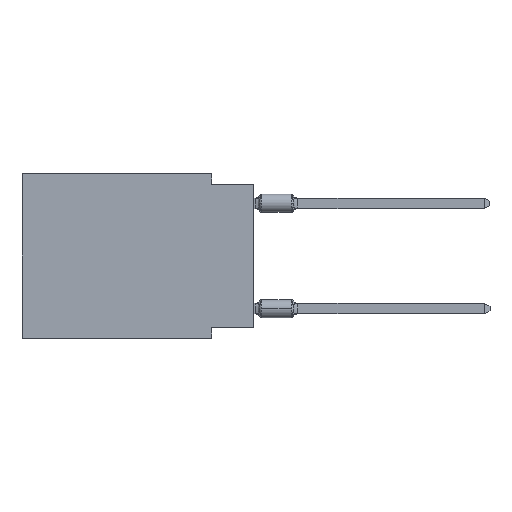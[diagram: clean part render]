
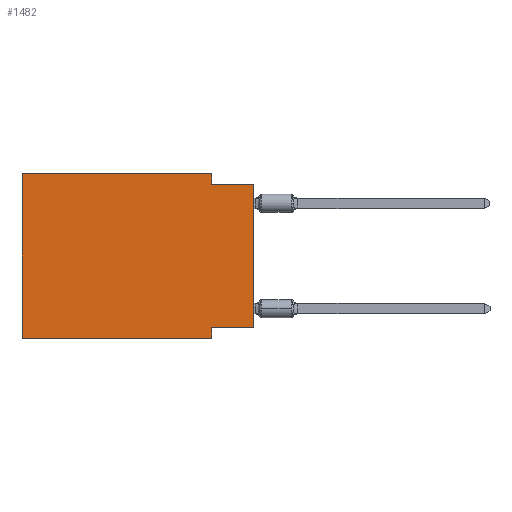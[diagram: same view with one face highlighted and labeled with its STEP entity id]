
A CAD part, left-side view. The second image highlights one B-rep face of the part: STEP entity #1482.
In plain terms, the highlighted planar face has unit normal (-1, 0, 0).
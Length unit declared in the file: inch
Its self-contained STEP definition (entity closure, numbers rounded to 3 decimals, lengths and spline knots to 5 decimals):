
#511 = DIRECTION ( 'NONE',  ( 0., 1., 0. ) ) ;
#536 = ORIENTED_EDGE ( 'NONE', *, *, #10044, .F. ) ;
#1262 = VERTEX_POINT ( 'NONE', #12577 ) ;
#1270 = CARTESIAN_POINT ( 'NONE',  ( 0., 0.55, 0. ) ) ;
#1482 = ADVANCED_FACE ( 'NONE', ( #9020 ), #8952, .F. ) ;
#1537 = CARTESIAN_POINT ( 'NONE',  ( 0., 0., -0.025 ) ) ;
#1590 = CARTESIAN_POINT ( 'NONE',  ( 0., 0.55, -0.39 ) ) ;
#1946 = ORIENTED_EDGE ( 'NONE', *, *, #8551, .F. ) ;
#2027 = ORIENTED_EDGE ( 'NONE', *, *, #4005, .F. ) ;
#2389 = CARTESIAN_POINT ( 'NONE',  ( 0., 0.1, -0.365 ) ) ;
#2416 = CARTESIAN_POINT ( 'NONE',  ( 0., 0., -0.365 ) ) ;
#2863 = CARTESIAN_POINT ( 'NONE',  ( 0., 0.55, 0. ) ) ;
#2995 = CARTESIAN_POINT ( 'NONE',  ( 0., 0.55, 0. ) ) ;
#3547 = LINE ( 'NONE', #4479, #10289 ) ;
#3612 = VECTOR ( 'NONE', #3818, 39.37008 ) ;
#3723 = ORIENTED_EDGE ( 'NONE', *, *, #9198, .F. ) ;
#3733 = VECTOR ( 'NONE', #7830, 39.37008 ) ;
#3818 = DIRECTION ( 'NONE',  ( 0., 0., -1. ) ) ;
#3841 = CARTESIAN_POINT ( 'NONE',  ( 0., 0.1, 0. ) ) ;
#3876 = LINE ( 'NONE', #5718, #3612 ) ;
#4005 = EDGE_CURVE ( 'NONE', #7941, #4395, #8879, .T. ) ;
#4129 = CARTESIAN_POINT ( 'NONE',  ( 0., 0.1, -0.025 ) ) ;
#4296 = EDGE_CURVE ( 'NONE', #4395, #7057, #8534, .T. ) ;
#4395 = VERTEX_POINT ( 'NONE', #4129 ) ;
#4479 = CARTESIAN_POINT ( 'NONE',  ( 0., 0.55, -0.39 ) ) ;
#4732 = DIRECTION ( 'NONE',  ( 0., -1., 0. ) ) ;
#4762 = CARTESIAN_POINT ( 'NONE',  ( 0., 0., 0. ) ) ;
#4778 = EDGE_LOOP ( 'NONE', ( #12218, #7010, #2027, #1946, #3723, #9507, #536, #12833 ) ) ;
#5616 = CARTESIAN_POINT ( 'NONE',  ( 0., 0., -0.365 ) ) ;
#5718 = CARTESIAN_POINT ( 'NONE',  ( 0., 0.1, -0.39 ) ) ;
#5893 = EDGE_CURVE ( 'NONE', #9913, #5908, #3547, .T. ) ;
#5908 = VERTEX_POINT ( 'NONE', #9576 ) ;
#5978 = VECTOR ( 'NONE', #6386, 39.37008 ) ;
#6138 = DIRECTION ( 'NONE',  ( 1., 0., 0. ) ) ;
#6309 = LINE ( 'NONE', #1270, #6315 ) ;
#6315 = VECTOR ( 'NONE', #7240, 39.37008 ) ;
#6386 = DIRECTION ( 'NONE',  ( 0., -1., 0. ) ) ;
#6786 = EDGE_CURVE ( 'NONE', #11885, #7057, #6987, .T. ) ;
#6987 = LINE ( 'NONE', #4762, #3733 ) ;
#6997 = DIRECTION ( 'NONE',  ( 0., 0., -1. ) ) ;
#7010 = ORIENTED_EDGE ( 'NONE', *, *, #4296, .F. ) ;
#7057 = VERTEX_POINT ( 'NONE', #8353 ) ;
#7240 = DIRECTION ( 'NONE',  ( 0., -1., 0. ) ) ;
#7774 = CARTESIAN_POINT ( 'NONE',  ( 0., 0.1, 0. ) ) ;
#7830 = DIRECTION ( 'NONE',  ( 0., 0., 1. ) ) ;
#7884 = EDGE_CURVE ( 'NONE', #11885, #11013, #9682, .T. ) ;
#7902 = LINE ( 'NONE', #2863, #11966 ) ;
#7941 = VERTEX_POINT ( 'NONE', #7774 ) ;
#8353 = CARTESIAN_POINT ( 'NONE',  ( 0., 0., -0.025 ) ) ;
#8534 = LINE ( 'NONE', #1537, #5978 ) ;
#8551 = EDGE_CURVE ( 'NONE', #1262, #7941, #6309, .T. ) ;
#8818 = DIRECTION ( 'NONE',  ( 0., 0., 1. ) ) ;
#8879 = LINE ( 'NONE', #3841, #12903 ) ;
#8952 = PLANE ( 'NONE',  #10871 ) ;
#9020 = FACE_OUTER_BOUND ( 'NONE', #4778, .T. ) ;
#9198 = EDGE_CURVE ( 'NONE', #9913, #1262, #7902, .T. ) ;
#9507 = ORIENTED_EDGE ( 'NONE', *, *, #5893, .T. ) ;
#9576 = CARTESIAN_POINT ( 'NONE',  ( 0., 0.1, -0.39 ) ) ;
#9682 = LINE ( 'NONE', #5616, #11502 ) ;
#9913 = VERTEX_POINT ( 'NONE', #1590 ) ;
#10044 = EDGE_CURVE ( 'NONE', #11013, #5908, #3876, .T. ) ;
#10289 = VECTOR ( 'NONE', #4732, 39.37008 ) ;
#10871 = AXIS2_PLACEMENT_3D ( 'NONE', #2995, #6138, #6997 ) ;
#11013 = VERTEX_POINT ( 'NONE', #2389 ) ;
#11502 = VECTOR ( 'NONE', #511, 39.37008 ) ;
#11885 = VERTEX_POINT ( 'NONE', #2416 ) ;
#11966 = VECTOR ( 'NONE', #8818, 39.37008 ) ;
#12218 = ORIENTED_EDGE ( 'NONE', *, *, #6786, .T. ) ;
#12577 = CARTESIAN_POINT ( 'NONE',  ( 0., 0.55, 0. ) ) ;
#12833 = ORIENTED_EDGE ( 'NONE', *, *, #7884, .F. ) ;
#12888 = DIRECTION ( 'NONE',  ( 0., 0., -1. ) ) ;
#12903 = VECTOR ( 'NONE', #12888, 39.37008 ) ;
